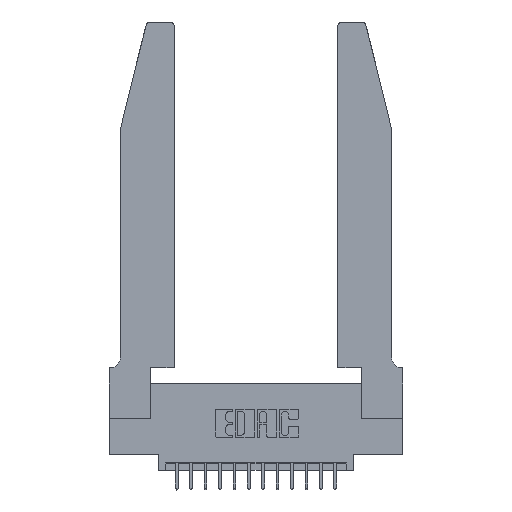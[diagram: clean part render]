
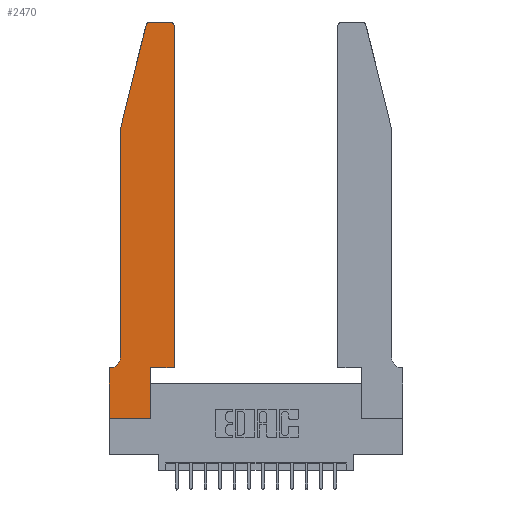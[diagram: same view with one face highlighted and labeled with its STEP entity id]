
A CAD part, top view. The second image highlights one B-rep face of the part: STEP entity #2470.
In plain terms, the highlighted planar face has unit normal (0, 0, 1).
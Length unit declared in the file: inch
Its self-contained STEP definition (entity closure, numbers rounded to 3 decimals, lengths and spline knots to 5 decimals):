
#95 = EDGE_CURVE ( 'NONE', #18345, #6549, #17370, .T. ) ;
#410 = DIRECTION ( 'NONE',  ( 0., 0., 1. ) ) ;
#516 = DIRECTION ( 'NONE',  ( 0., -1., 0. ) ) ;
#655 = EDGE_LOOP ( 'NONE', ( #918, #5624, #12937, #8281, #5215, #6477, #9454, #14268, #3562, #16129, #12284, #861 ) ) ;
#861 = ORIENTED_EDGE ( 'NONE', *, *, #9329, .T. ) ;
#918 = ORIENTED_EDGE ( 'NONE', *, *, #1102, .T. ) ;
#1102 = EDGE_CURVE ( 'NONE', #13299, #10712, #13859, .T. ) ;
#1459 = VECTOR ( 'NONE', #516, 39.37008 ) ;
#1644 = CARTESIAN_POINT ( 'NONE',  ( 0.4505, 0.35, 0.37 ) ) ;
#1710 = CARTESIAN_POINT ( 'NONE',  ( 0.0755, 2., 0.37 ) ) ;
#2000 = LINE ( 'NONE', #17395, #1459 ) ;
#2150 = DIRECTION ( 'NONE',  ( 1., 0., 0. ) ) ;
#2268 = CARTESIAN_POINT ( 'NONE',  ( 0.4505, 2.72, 0.37 ) ) ;
#2470 = ADVANCED_FACE ( 'NONE', ( #8228 ), #9611, .T. ) ;
#3329 = VECTOR ( 'NONE', #10182, 39.37008 ) ;
#3562 = ORIENTED_EDGE ( 'NONE', *, *, #10957, .T. ) ;
#3701 = EDGE_CURVE ( 'NONE', #3867, #7758, #17708, .T. ) ;
#3820 = VERTEX_POINT ( 'NONE', #5690 ) ;
#3867 = VERTEX_POINT ( 'NONE', #6146 ) ;
#3984 = VECTOR ( 'NONE', #16087, 39.37008 ) ;
#4605 = LINE ( 'NONE', #18403, #12509 ) ;
#4656 = DIRECTION ( 'NONE',  ( 1., 0., 0. ) ) ;
#4727 = CARTESIAN_POINT ( 'NONE',  ( 0.2865, 0.35, 0.37 ) ) ;
#4968 = CARTESIAN_POINT ( 'NONE',  ( 0.0755, 0.35, 0.37 ) ) ;
#5134 = CARTESIAN_POINT ( 'NONE',  ( 0.4505, 0.35, 0.37 ) ) ;
#5215 = ORIENTED_EDGE ( 'NONE', *, *, #7207, .T. ) ;
#5539 = VERTEX_POINT ( 'NONE', #12664 ) ;
#5624 = ORIENTED_EDGE ( 'NONE', *, *, #9946, .T. ) ;
#5690 = CARTESIAN_POINT ( 'NONE',  ( 0., 0., 0.37 ) ) ;
#5891 = CIRCLE ( 'NONE', #11829, 0.03 ) ;
#5930 = CARTESIAN_POINT ( 'NONE',  ( 0.284, 2.75, 0.37 ) ) ;
#6146 = CARTESIAN_POINT ( 'NONE',  ( 0.0055, 0.35, 0.37 ) ) ;
#6477 = ORIENTED_EDGE ( 'NONE', *, *, #3701, .T. ) ;
#6549 = VERTEX_POINT ( 'NONE', #17413 ) ;
#6613 = VERTEX_POINT ( 'NONE', #5134 ) ;
#6664 = VERTEX_POINT ( 'NONE', #10818 ) ;
#6828 = DIRECTION ( 'NONE',  ( 1., 0., 0. ) ) ;
#6842 = CARTESIAN_POINT ( 'NONE',  ( 0., 0., 0.37 ) ) ;
#7165 = EDGE_CURVE ( 'NONE', #7758, #3820, #14256, .T. ) ;
#7207 = EDGE_CURVE ( 'NONE', #6664, #3867, #13569, .T. ) ;
#7301 = CARTESIAN_POINT ( 'NONE',  ( 0.0055, 0.42, 0.37 ) ) ;
#7313 = CARTESIAN_POINT ( 'NONE',  ( 0.25487, 2.72718, 0.37 ) ) ;
#7758 = VERTEX_POINT ( 'NONE', #14279 ) ;
#8228 = FACE_OUTER_BOUND ( 'NONE', #655, .T. ) ;
#8281 = ORIENTED_EDGE ( 'NONE', *, *, #13460, .T. ) ;
#8323 = DIRECTION ( 'NONE',  ( 0., 0., 1. ) ) ;
#8557 = AXIS2_PLACEMENT_3D ( 'NONE', #7301, #10169, #12945 ) ;
#8605 = AXIS2_PLACEMENT_3D ( 'NONE', #15377, #8323, #6828 ) ;
#8846 = VERTEX_POINT ( 'NONE', #2268 ) ;
#9329 = EDGE_CURVE ( 'NONE', #8846, #13299, #10337, .T. ) ;
#9386 = VECTOR ( 'NONE', #14625, 39.37008 ) ;
#9454 = ORIENTED_EDGE ( 'NONE', *, *, #7165, .T. ) ;
#9611 = PLANE ( 'NONE',  #8605 ) ;
#9946 = EDGE_CURVE ( 'NONE', #10712, #18345, #5891, .T. ) ;
#10169 = DIRECTION ( 'NONE',  ( 0., 0., -1. ) ) ;
#10182 = DIRECTION ( 'NONE',  ( 1., 0., 0. ) ) ;
#10308 = DIRECTION ( 'NONE',  ( 0., 1., 0. ) ) ;
#10337 = CIRCLE ( 'NONE', #17446, 0.03 ) ;
#10712 = VERTEX_POINT ( 'NONE', #5930 ) ;
#10818 = CARTESIAN_POINT ( 'NONE',  ( 0.0755, 0.42, 0.37 ) ) ;
#10957 = EDGE_CURVE ( 'NONE', #18263, #5539, #11801, .T. ) ;
#11731 = CARTESIAN_POINT ( 'NONE',  ( 0.284, 2.72, 0.37 ) ) ;
#11794 = DIRECTION ( 'NONE',  ( 0., 0., 1. ) ) ;
#11801 = LINE ( 'NONE', #4727, #16304 ) ;
#11829 = AXIS2_PLACEMENT_3D ( 'NONE', #11731, #410, #14327 ) ;
#12225 = DIRECTION ( 'NONE',  ( -1., 0., 0. ) ) ;
#12284 = ORIENTED_EDGE ( 'NONE', *, *, #13805, .T. ) ;
#12509 = VECTOR ( 'NONE', #10308, 39.37008 ) ;
#12664 = CARTESIAN_POINT ( 'NONE',  ( 0.2865, 0.35, 0.37 ) ) ;
#12937 = ORIENTED_EDGE ( 'NONE', *, *, #95, .T. ) ;
#12945 = DIRECTION ( 'NONE',  ( -1., 0., 0. ) ) ;
#13299 = VERTEX_POINT ( 'NONE', #13776 ) ;
#13460 = EDGE_CURVE ( 'NONE', #6549, #6664, #2000, .T. ) ;
#13523 = EDGE_CURVE ( 'NONE', #5539, #6613, #15925, .T. ) ;
#13569 = CIRCLE ( 'NONE', #8557, 0.07 ) ;
#13776 = CARTESIAN_POINT ( 'NONE',  ( 0.4205, 2.75, 0.37 ) ) ;
#13805 = EDGE_CURVE ( 'NONE', #6613, #8846, #4605, .T. ) ;
#13859 = LINE ( 'NONE', #16292, #17111 ) ;
#13897 = LINE ( 'NONE', #6842, #3329 ) ;
#14081 = CARTESIAN_POINT ( 'NONE',  ( 0.2865, 0., 0.37 ) ) ;
#14256 = LINE ( 'NONE', #14438, #9386 ) ;
#14268 = ORIENTED_EDGE ( 'NONE', *, *, #18219, .T. ) ;
#14279 = CARTESIAN_POINT ( 'NONE',  ( 0., 0.35, 0.37 ) ) ;
#14327 = DIRECTION ( 'NONE',  ( 1., 0., 0. ) ) ;
#14438 = CARTESIAN_POINT ( 'NONE',  ( 0., 0., 0.37 ) ) ;
#14625 = DIRECTION ( 'NONE',  ( 0., -1., 0. ) ) ;
#15377 = CARTESIAN_POINT ( 'NONE',  ( 0., 0.35, 0.37 ) ) ;
#15925 = LINE ( 'NONE', #1644, #16652 ) ;
#16087 = DIRECTION ( 'NONE',  ( -0.239, -0.971, 0. ) ) ;
#16129 = ORIENTED_EDGE ( 'NONE', *, *, #13523, .T. ) ;
#16292 = CARTESIAN_POINT ( 'NONE',  ( 0.2605, 2.75, 0.37 ) ) ;
#16304 = VECTOR ( 'NONE', #17739, 39.37008 ) ;
#16560 = DIRECTION ( 'NONE',  ( -1., 0., 0. ) ) ;
#16652 = VECTOR ( 'NONE', #4656, 39.37008 ) ;
#17111 = VECTOR ( 'NONE', #16560, 39.37008 ) ;
#17341 = VECTOR ( 'NONE', #12225, 39.37008 ) ;
#17370 = LINE ( 'NONE', #1710, #3984 ) ;
#17395 = CARTESIAN_POINT ( 'NONE',  ( 0.0755, 2., 0.37 ) ) ;
#17413 = CARTESIAN_POINT ( 'NONE',  ( 0.0755, 2., 0.37 ) ) ;
#17446 = AXIS2_PLACEMENT_3D ( 'NONE', #17637, #11794, #2150 ) ;
#17637 = CARTESIAN_POINT ( 'NONE',  ( 0.4205, 2.72, 0.37 ) ) ;
#17708 = LINE ( 'NONE', #4968, #17341 ) ;
#17739 = DIRECTION ( 'NONE',  ( 0., 1., 0. ) ) ;
#18219 = EDGE_CURVE ( 'NONE', #3820, #18263, #13897, .T. ) ;
#18263 = VERTEX_POINT ( 'NONE', #14081 ) ;
#18345 = VERTEX_POINT ( 'NONE', #7313 ) ;
#18403 = CARTESIAN_POINT ( 'NONE',  ( 0.4505, 0.35, 0.37 ) ) ;
